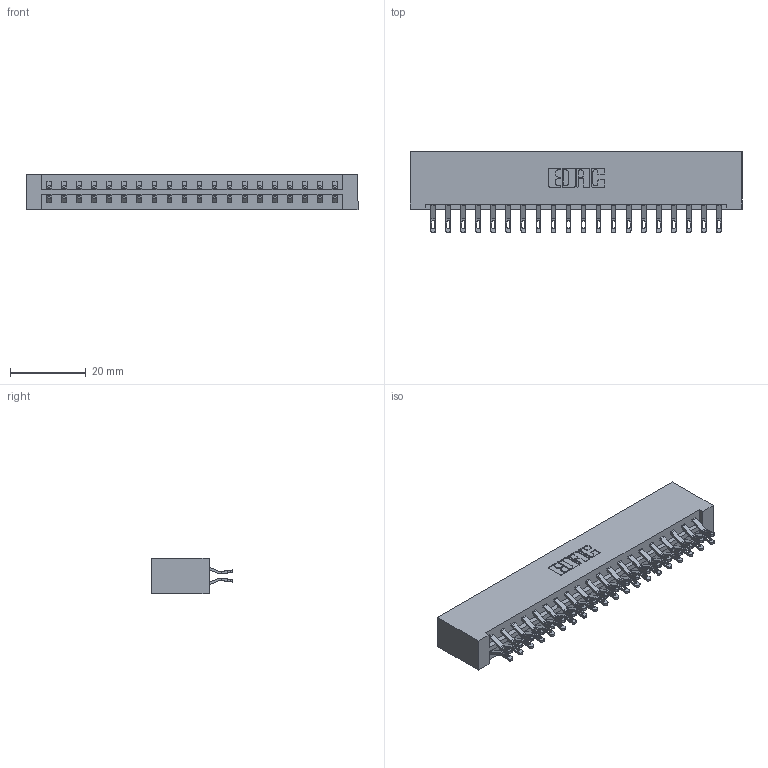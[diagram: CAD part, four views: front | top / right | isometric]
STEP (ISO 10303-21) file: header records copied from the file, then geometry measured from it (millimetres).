
FILE_DESCRIPTION (( 'STEP AP203' ), '1' );
FILE_NAME ('333-040-555-201.STEP', '2018-08-03T14:33:43', ( '' ), ( '' ), 'SwSTEP 2.0', 'SolidWorks 2016', '' );
FILE_SCHEMA (( 'CONFIG_CONTROL_DESIGN' ));
Length unit declared in the file: inch
Products named in the file (3): 333 Part_Lugless; 345-292-001_555 Tail; 333-040-555-201
Assembly tree (41 placements, depth 2):
  333-040-555-201
    333 Part_Lugless
    345-292-001_555 Tail  x40
Bounding box: 87.5 x 21.47 x 9.4 mm (x, y, z)
Volume: 9476.1 mm3; surface area: 11424.9 mm2
Topology: 41 solids, 41 shells, 2426 faces, 7607 edges, 5070 vertices
Faces by surface type: plane 1426, cylinder 1000
Entity records: 15761 total; most frequent: CARTESIAN_POINT 2672, ORIENTED_EDGE 2578, DIRECTION 2285, EDGE_CURVE 1289, LINE 1149, VECTOR 1149, VERTEX_POINT 858, AXIS2_PLACEMENT_3D 568
